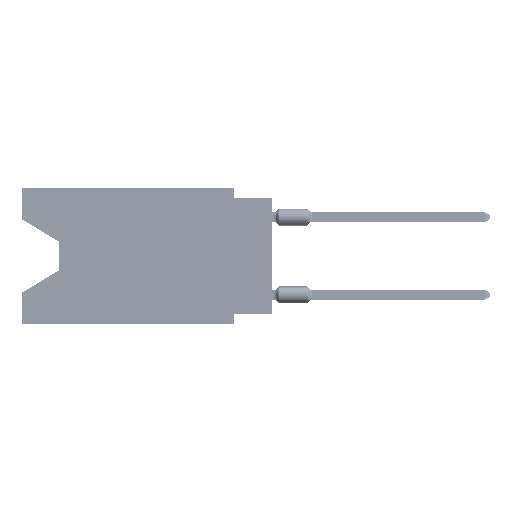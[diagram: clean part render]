
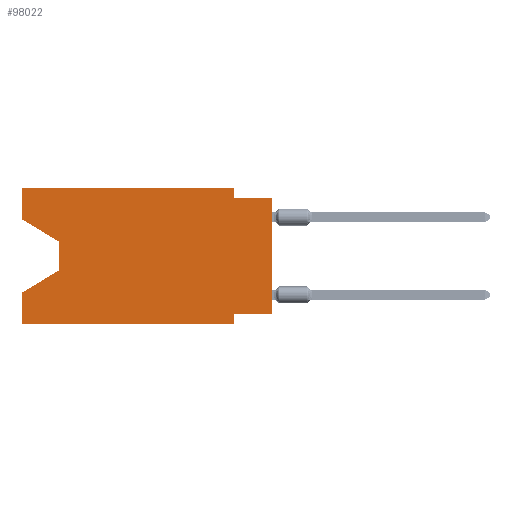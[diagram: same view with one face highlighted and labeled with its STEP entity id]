
A CAD part, left-side view. The second image highlights one B-rep face of the part: STEP entity #98022.
In plain terms, the highlighted planar face has unit normal (-1, 0, 0).
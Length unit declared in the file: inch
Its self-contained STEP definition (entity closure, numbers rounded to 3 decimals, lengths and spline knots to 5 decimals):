
#1246 = VECTOR ( 'NONE', #96211, 39.37008 ) ;
#2509 = EDGE_CURVE ( 'NONE', #47234, #58905, #14464, .T. ) ;
#2628 = CARTESIAN_POINT ( 'NONE',  ( 0., 0.645, 0. ) ) ;
#4859 = LINE ( 'NONE', #37668, #82374 ) ;
#6674 = ORIENTED_EDGE ( 'NONE', *, *, #81840, .F. ) ;
#7103 = CARTESIAN_POINT ( 'NONE',  ( 0., 0.645, -0.35 ) ) ;
#7252 = LINE ( 'NONE', #83066, #86551 ) ;
#7626 = CARTESIAN_POINT ( 'NONE',  ( 0., 0.55, -0.212 ) ) ;
#9816 = EDGE_CURVE ( 'NONE', #64604, #18273, #46574, .T. ) ;
#10656 = PLANE ( 'NONE',  #72446 ) ;
#10882 = DIRECTION ( 'NONE',  ( 0., -0.855, -0.519 ) ) ;
#11957 = EDGE_CURVE ( 'NONE', #33256, #67408, #7252, .T. ) ;
#12055 = LINE ( 'NONE', #28777, #20740 ) ;
#13869 = LINE ( 'NONE', #69844, #19234 ) ;
#14464 = LINE ( 'NONE', #80109, #1246 ) ;
#15229 = VERTEX_POINT ( 'NONE', #71216 ) ;
#15368 = DIRECTION ( 'NONE',  ( 0., 1., 0. ) ) ;
#15588 = VECTOR ( 'NONE', #89813, 39.37008 ) ;
#15872 = DIRECTION ( 'NONE',  ( 0., 0.855, -0.519 ) ) ;
#16360 = CARTESIAN_POINT ( 'NONE',  ( 0., 0., -0.325 ) ) ;
#16576 = VECTOR ( 'NONE', #49841, 39.37008 ) ;
#17173 = FACE_OUTER_BOUND ( 'NONE', #47767, .T. ) ;
#17873 = CARTESIAN_POINT ( 'NONE',  ( 0., 0.645, -0.08025 ) ) ;
#18269 = LINE ( 'NONE', #25800, #15588 ) ;
#18273 = VERTEX_POINT ( 'NONE', #50563 ) ;
#19131 = ORIENTED_EDGE ( 'NONE', *, *, #9816, .F. ) ;
#19234 = VECTOR ( 'NONE', #45084, 39.37008 ) ;
#20740 = VECTOR ( 'NONE', #84691, 39.37008 ) ;
#21841 = CARTESIAN_POINT ( 'NONE',  ( 0., 0., -0.025 ) ) ;
#22104 = ORIENTED_EDGE ( 'NONE', *, *, #38827, .T. ) ;
#22365 = CARTESIAN_POINT ( 'NONE',  ( 0., 0.645, -0.35 ) ) ;
#22411 = VERTEX_POINT ( 'NONE', #21841 ) ;
#23246 = VECTOR ( 'NONE', #15368, 39.37008 ) ;
#23289 = LINE ( 'NONE', #7103, #48738 ) ;
#23698 = VECTOR ( 'NONE', #64366, 39.37008 ) ;
#25800 = CARTESIAN_POINT ( 'NONE',  ( 0., 0.55, -0.138 ) ) ;
#26833 = CARTESIAN_POINT ( 'NONE',  ( 0., 0.1, -0.35 ) ) ;
#28478 = DIRECTION ( 'NONE',  ( 0., 0., 1. ) ) ;
#28777 = CARTESIAN_POINT ( 'NONE',  ( 0., 0.645, 0. ) ) ;
#28893 = ORIENTED_EDGE ( 'NONE', *, *, #42425, .F. ) ;
#32793 = VECTOR ( 'NONE', #28478, 39.37008 ) ;
#33256 = VERTEX_POINT ( 'NONE', #7626 ) ;
#34897 = DIRECTION ( 'NONE',  ( 1., 0., 0. ) ) ;
#35046 = ORIENTED_EDGE ( 'NONE', *, *, #48861, .F. ) ;
#37281 = VECTOR ( 'NONE', #10882, 39.37008 ) ;
#37668 = CARTESIAN_POINT ( 'NONE',  ( 0., 0.1, 0. ) ) ;
#38717 = EDGE_CURVE ( 'NONE', #56491, #33256, #18269, .T. ) ;
#38827 = EDGE_CURVE ( 'NONE', #64604, #22411, #92980, .T. ) ;
#42156 = ORIENTED_EDGE ( 'NONE', *, *, #44220, .T. ) ;
#42425 = EDGE_CURVE ( 'NONE', #15229, #22411, #13869, .T. ) ;
#44054 = CARTESIAN_POINT ( 'NONE',  ( 0., 0., 0. ) ) ;
#44220 = EDGE_CURVE ( 'NONE', #45515, #96372, #23289, .T. ) ;
#45084 = DIRECTION ( 'NONE',  ( 0., -1., 0. ) ) ;
#45226 = ORIENTED_EDGE ( 'NONE', *, *, #2509, .F. ) ;
#45515 = VERTEX_POINT ( 'NONE', #22365 ) ;
#46381 = CARTESIAN_POINT ( 'NONE',  ( 0., 0.645, 0. ) ) ;
#46574 = LINE ( 'NONE', #72926, #23246 ) ;
#47234 = VERTEX_POINT ( 'NONE', #17873 ) ;
#47767 = EDGE_LOOP ( 'NONE', ( #87964, #105253, #76496, #35046, #42156, #6674, #19131, #22104, #28893, #104661, #53893, #45226 ) ) ;
#48738 = VECTOR ( 'NONE', #96414, 39.37008 ) ;
#48861 = EDGE_CURVE ( 'NONE', #45515, #67408, #106331, .T. ) ;
#49841 = DIRECTION ( 'NONE',  ( 0., 0., 1. ) ) ;
#50563 = CARTESIAN_POINT ( 'NONE',  ( 0., 0.1, -0.325 ) ) ;
#52720 = EDGE_CURVE ( 'NONE', #95067, #15229, #4859, .T. ) ;
#53893 = ORIENTED_EDGE ( 'NONE', *, *, #85483, .F. ) ;
#56287 = CARTESIAN_POINT ( 'NONE',  ( 0., 0.1, -0.35 ) ) ;
#56491 = VERTEX_POINT ( 'NONE', #59031 ) ;
#58767 = CARTESIAN_POINT ( 'NONE',  ( 0., 0.645, -0.08025 ) ) ;
#58905 = VERTEX_POINT ( 'NONE', #46381 ) ;
#59031 = CARTESIAN_POINT ( 'NONE',  ( 0., 0.55, -0.138 ) ) ;
#64366 = DIRECTION ( 'NONE',  ( 0., 0., -1. ) ) ;
#64604 = VERTEX_POINT ( 'NONE', #16360 ) ;
#64737 = EDGE_CURVE ( 'NONE', #47234, #56491, #84590, .T. ) ;
#65128 = CARTESIAN_POINT ( 'NONE',  ( 0., 0.645, -0.26975 ) ) ;
#67408 = VERTEX_POINT ( 'NONE', #65128 ) ;
#67703 = DIRECTION ( 'NONE',  ( 0., 0., -1. ) ) ;
#69844 = CARTESIAN_POINT ( 'NONE',  ( 0., 0., -0.025 ) ) ;
#70464 = DIRECTION ( 'NONE',  ( 0., 0., -1. ) ) ;
#71216 = CARTESIAN_POINT ( 'NONE',  ( 0., 0.1, -0.025 ) ) ;
#72446 = AXIS2_PLACEMENT_3D ( 'NONE', #2628, #34897, #67703 ) ;
#72926 = CARTESIAN_POINT ( 'NONE',  ( 0., 0., -0.325 ) ) ;
#76496 = ORIENTED_EDGE ( 'NONE', *, *, #11957, .T. ) ;
#78790 = CARTESIAN_POINT ( 'NONE',  ( 0., 0.1, 0. ) ) ;
#80109 = CARTESIAN_POINT ( 'NONE',  ( 0., 0.645, 0. ) ) ;
#81840 = EDGE_CURVE ( 'NONE', #18273, #96372, #106298, .T. ) ;
#82374 = VECTOR ( 'NONE', #70464, 39.37008 ) ;
#83066 = CARTESIAN_POINT ( 'NONE',  ( 0., 0.55, -0.212 ) ) ;
#84590 = LINE ( 'NONE', #58767, #37281 ) ;
#84691 = DIRECTION ( 'NONE',  ( 0., -1., 0. ) ) ;
#85483 = EDGE_CURVE ( 'NONE', #58905, #95067, #12055, .T. ) ;
#86551 = VECTOR ( 'NONE', #15872, 39.37008 ) ;
#87964 = ORIENTED_EDGE ( 'NONE', *, *, #64737, .T. ) ;
#89660 = CARTESIAN_POINT ( 'NONE',  ( 0., 0.645, 0. ) ) ;
#89813 = DIRECTION ( 'NONE',  ( 0., 0., -1. ) ) ;
#92980 = LINE ( 'NONE', #44054, #32793 ) ;
#95067 = VERTEX_POINT ( 'NONE', #78790 ) ;
#96211 = DIRECTION ( 'NONE',  ( 0., 0., 1. ) ) ;
#96372 = VERTEX_POINT ( 'NONE', #26833 ) ;
#96414 = DIRECTION ( 'NONE',  ( 0., -1., 0. ) ) ;
#98022 = ADVANCED_FACE ( 'NONE', ( #17173 ), #10656, .F. ) ;
#104661 = ORIENTED_EDGE ( 'NONE', *, *, #52720, .F. ) ;
#105253 = ORIENTED_EDGE ( 'NONE', *, *, #38717, .T. ) ;
#106298 = LINE ( 'NONE', #56287, #23698 ) ;
#106331 = LINE ( 'NONE', #89660, #16576 ) ;
